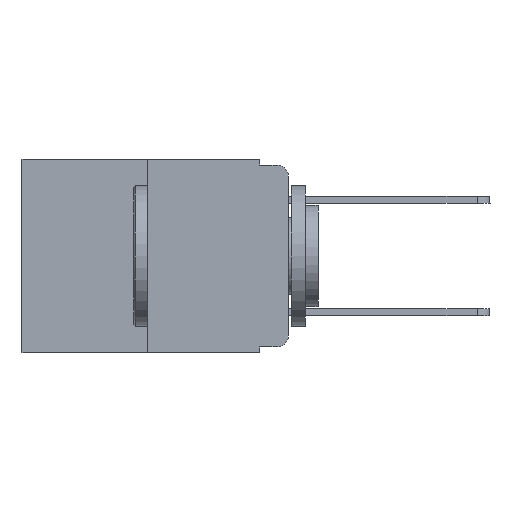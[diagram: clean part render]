
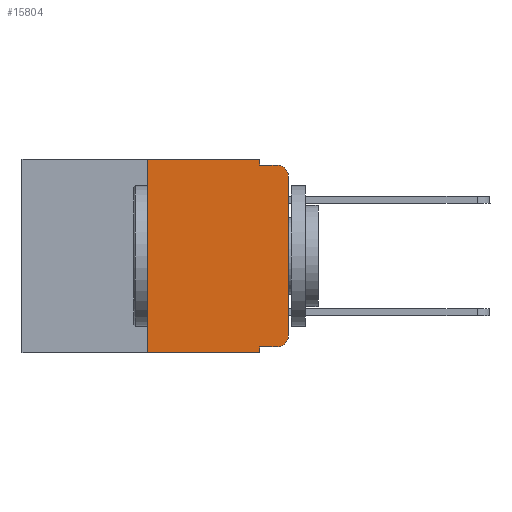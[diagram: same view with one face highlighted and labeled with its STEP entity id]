
A CAD part, left-side view. The second image highlights one B-rep face of the part: STEP entity #15804.
In plain terms, the highlighted planar face has unit normal (-1, 0, 0).
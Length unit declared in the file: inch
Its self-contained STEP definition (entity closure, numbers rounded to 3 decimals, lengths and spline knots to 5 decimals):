
#644 = VERTEX_POINT ( 'NONE', #2034 ) ;
#718 = EDGE_CURVE ( 'NONE', #18341, #11641, #10087, .T. ) ;
#1102 = VECTOR ( 'NONE', #12207, 39.37008 ) ;
#1316 = CARTESIAN_POINT ( 'NONE',  ( 0., 0.473, -0.343 ) ) ;
#1375 = LINE ( 'NONE', #7537, #1102 ) ;
#1768 = CARTESIAN_POINT ( 'NONE',  ( 0., 0.051, -0.01 ) ) ;
#1834 = PLANE ( 'NONE',  #7800 ) ;
#1945 = VERTEX_POINT ( 'NONE', #15933 ) ;
#2034 = CARTESIAN_POINT ( 'NONE',  ( 0., 0., -0.03 ) ) ;
#2225 = CARTESIAN_POINT ( 'NONE',  ( 0., 0.25, 0. ) ) ;
#2749 = ORIENTED_EDGE ( 'NONE', *, *, #8529, .T. ) ;
#3096 = DIRECTION ( 'NONE',  ( 0., -1., 0. ) ) ;
#3404 = ORIENTED_EDGE ( 'NONE', *, *, #7994, .T. ) ;
#4090 = VERTEX_POINT ( 'NONE', #17816 ) ;
#4221 = CARTESIAN_POINT ( 'NONE',  ( 0., 0.051, 0. ) ) ;
#4239 = CARTESIAN_POINT ( 'NONE',  ( 0., 0.051, -0.333 ) ) ;
#5261 = DIRECTION ( 'NONE',  ( -1., 0., 0. ) ) ;
#5391 = CARTESIAN_POINT ( 'NONE',  ( 0., 0.02, -0.03 ) ) ;
#5626 = ORIENTED_EDGE ( 'NONE', *, *, #11819, .T. ) ;
#5993 = VERTEX_POINT ( 'NONE', #7534 ) ;
#6069 = DIRECTION ( 'NONE',  ( 0., -1., 0. ) ) ;
#6365 = VECTOR ( 'NONE', #16150, 39.37008 ) ;
#6821 = VECTOR ( 'NONE', #7291, 39.37008 ) ;
#6964 = AXIS2_PLACEMENT_3D ( 'NONE', #19159, #5261, #11436 ) ;
#7083 = DIRECTION ( 'NONE',  ( 0., 0., -1. ) ) ;
#7291 = DIRECTION ( 'NONE',  ( 0., -1., 0. ) ) ;
#7452 = CARTESIAN_POINT ( 'NONE',  ( 0., 0.02, -0.333 ) ) ;
#7487 = EDGE_CURVE ( 'NONE', #5993, #17707, #1375, .T. ) ;
#7525 = EDGE_CURVE ( 'NONE', #1945, #5993, #12608, .T. ) ;
#7534 = CARTESIAN_POINT ( 'NONE',  ( 0., 0.051, 0. ) ) ;
#7537 = CARTESIAN_POINT ( 'NONE',  ( 0., 0.051, 0. ) ) ;
#7800 = AXIS2_PLACEMENT_3D ( 'NONE', #9111, #15292, #15397 ) ;
#7994 = EDGE_CURVE ( 'NONE', #4090, #11641, #17062, .T. ) ;
#8445 = VERTEX_POINT ( 'NONE', #7452 ) ;
#8529 = EDGE_CURVE ( 'NONE', #644, #18457, #14385, .T. ) ;
#9082 = EDGE_CURVE ( 'NONE', #8445, #11396, #15036, .T. ) ;
#9111 = CARTESIAN_POINT ( 'NONE',  ( 0., 0.473, 0. ) ) ;
#9141 = ORIENTED_EDGE ( 'NONE', *, *, #16964, .F. ) ;
#9303 = ORIENTED_EDGE ( 'NONE', *, *, #15726, .T. ) ;
#10087 = LINE ( 'NONE', #4221, #19197 ) ;
#10457 = VECTOR ( 'NONE', #6069, 39.37008 ) ;
#11083 = EDGE_LOOP ( 'NONE', ( #5626, #2749, #9141, #17793, #17336, #18421, #3404, #12465, #9303, #12864 ) ) ;
#11396 = VERTEX_POINT ( 'NONE', #17703 ) ;
#11418 = LINE ( 'NONE', #2225, #18796 ) ;
#11436 = DIRECTION ( 'NONE',  ( 0., 0., -1. ) ) ;
#11440 = VECTOR ( 'NONE', #3096, 39.37008 ) ;
#11579 = CARTESIAN_POINT ( 'NONE',  ( 0., 0., 0. ) ) ;
#11641 = VERTEX_POINT ( 'NONE', #18493 ) ;
#11709 = LINE ( 'NONE', #13324, #13576 ) ;
#11713 = CARTESIAN_POINT ( 'NONE',  ( 0., 0.051, -0.333 ) ) ;
#11819 = EDGE_CURVE ( 'NONE', #11396, #644, #16342, .T. ) ;
#12053 = LINE ( 'NONE', #4239, #6821 ) ;
#12207 = DIRECTION ( 'NONE',  ( 0., 0., -1. ) ) ;
#12465 = ORIENTED_EDGE ( 'NONE', *, *, #718, .F. ) ;
#12608 = LINE ( 'NONE', #14325, #11440 ) ;
#12623 = DIRECTION ( 'NONE',  ( 0., 0., -1. ) ) ;
#12864 = ORIENTED_EDGE ( 'NONE', *, *, #9082, .T. ) ;
#13324 = CARTESIAN_POINT ( 'NONE',  ( 0., 0.051, -0.01 ) ) ;
#13576 = VECTOR ( 'NONE', #14944, 39.37008 ) ;
#14325 = CARTESIAN_POINT ( 'NONE',  ( 0., 0.473, 0. ) ) ;
#14385 = CIRCLE ( 'NONE', #16006, 0.02 ) ;
#14944 = DIRECTION ( 'NONE',  ( 0., -1., 0. ) ) ;
#15036 = CIRCLE ( 'NONE', #6964, 0.02 ) ;
#15292 = DIRECTION ( 'NONE',  ( 1., 0., 0. ) ) ;
#15397 = DIRECTION ( 'NONE',  ( 0., 0., -1. ) ) ;
#15703 = FACE_OUTER_BOUND ( 'NONE', #11083, .T. ) ;
#15726 = EDGE_CURVE ( 'NONE', #18341, #8445, #12053, .T. ) ;
#15804 = ADVANCED_FACE ( 'NONE', ( #15703 ), #1834, .F. ) ;
#15933 = CARTESIAN_POINT ( 'NONE',  ( 0., 0.25, 0. ) ) ;
#15997 = EDGE_CURVE ( 'NONE', #4090, #1945, #11418, .T. ) ;
#16006 = AXIS2_PLACEMENT_3D ( 'NONE', #5391, #17569, #12623 ) ;
#16150 = DIRECTION ( 'NONE',  ( 0., 0., 1. ) ) ;
#16342 = LINE ( 'NONE', #11579, #6365 ) ;
#16964 = EDGE_CURVE ( 'NONE', #17707, #18457, #11709, .T. ) ;
#17062 = LINE ( 'NONE', #1316, #10457 ) ;
#17336 = ORIENTED_EDGE ( 'NONE', *, *, #7525, .F. ) ;
#17535 = DIRECTION ( 'NONE',  ( 0., 0., 1. ) ) ;
#17569 = DIRECTION ( 'NONE',  ( -1., 0., 0. ) ) ;
#17703 = CARTESIAN_POINT ( 'NONE',  ( 0., 0., -0.313 ) ) ;
#17707 = VERTEX_POINT ( 'NONE', #1768 ) ;
#17793 = ORIENTED_EDGE ( 'NONE', *, *, #7487, .F. ) ;
#17816 = CARTESIAN_POINT ( 'NONE',  ( 0., 0.25, -0.343 ) ) ;
#18341 = VERTEX_POINT ( 'NONE', #11713 ) ;
#18421 = ORIENTED_EDGE ( 'NONE', *, *, #15997, .F. ) ;
#18457 = VERTEX_POINT ( 'NONE', #19106 ) ;
#18493 = CARTESIAN_POINT ( 'NONE',  ( 0., 0.051, -0.343 ) ) ;
#18796 = VECTOR ( 'NONE', #17535, 39.37008 ) ;
#19106 = CARTESIAN_POINT ( 'NONE',  ( 0., 0.02, -0.01 ) ) ;
#19159 = CARTESIAN_POINT ( 'NONE',  ( 0., 0.02, -0.313 ) ) ;
#19197 = VECTOR ( 'NONE', #7083, 39.37008 ) ;
